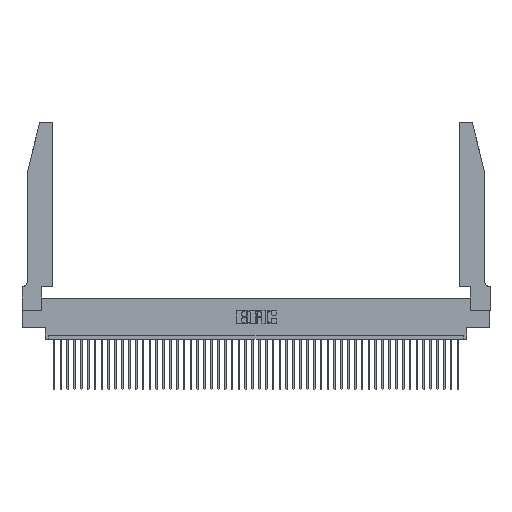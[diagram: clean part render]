
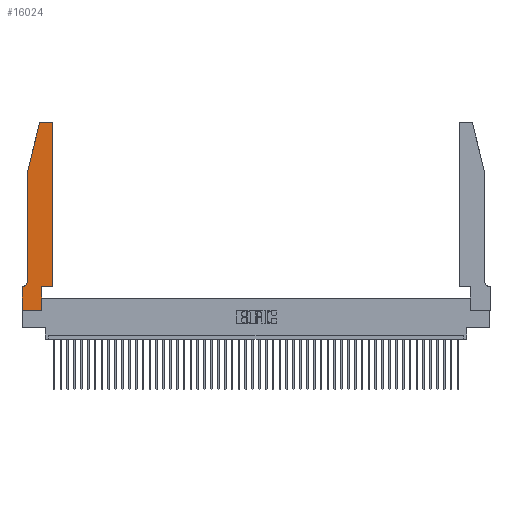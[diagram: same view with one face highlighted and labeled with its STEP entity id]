
A CAD part, top view. The second image highlights one B-rep face of the part: STEP entity #16024.
In plain terms, the highlighted planar face has unit normal (0, 0, 1).
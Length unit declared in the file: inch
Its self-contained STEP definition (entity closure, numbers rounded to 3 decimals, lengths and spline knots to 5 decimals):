
#218 = EDGE_CURVE ( 'NONE', #32804, #10812, #25990, .T. ) ;
#395 = VECTOR ( 'NONE', #32074, 39.37008 ) ;
#1540 = CARTESIAN_POINT ( 'NONE',  ( 0.284, 2.72, 0.37 ) ) ;
#2363 = VERTEX_POINT ( 'NONE', #44291 ) ;
#3165 = EDGE_CURVE ( 'NONE', #10812, #23474, #43766, .T. ) ;
#3370 = EDGE_CURVE ( 'NONE', #2363, #41579, #29880, .T. ) ;
#3627 = CARTESIAN_POINT ( 'NONE',  ( 0.2865, 0.35, 0.37 ) ) ;
#4248 = DIRECTION ( 'NONE',  ( 1., 0., 0. ) ) ;
#4582 = CARTESIAN_POINT ( 'NONE',  ( 0.4205, 2.72, 0.37 ) ) ;
#5202 = DIRECTION ( 'NONE',  ( 1., 0., 0. ) ) ;
#5893 = VECTOR ( 'NONE', #5202, 39.37008 ) ;
#6451 = LINE ( 'NONE', #23495, #5893 ) ;
#6571 = DIRECTION ( 'NONE',  ( 1., 0., 0. ) ) ;
#6599 = ORIENTED_EDGE ( 'NONE', *, *, #39795, .T. ) ;
#7477 = CARTESIAN_POINT ( 'NONE',  ( 0.0755, 0.35, 0.37 ) ) ;
#7932 = AXIS2_PLACEMENT_3D ( 'NONE', #4582, #29651, #4248 ) ;
#8199 = CIRCLE ( 'NONE', #40927, 0.03 ) ;
#8455 = ORIENTED_EDGE ( 'NONE', *, *, #41317, .T. ) ;
#9290 = DIRECTION ( 'NONE',  ( 0., 1., 0. ) ) ;
#9358 = VECTOR ( 'NONE', #35847, 39.37008 ) ;
#9424 = DIRECTION ( 'NONE',  ( 0., 0., -1. ) ) ;
#10183 = CARTESIAN_POINT ( 'NONE',  ( 0., 0., 0.37 ) ) ;
#10416 = DIRECTION ( 'NONE',  ( 0., 0., 1. ) ) ;
#10540 = CARTESIAN_POINT ( 'NONE',  ( 0.4505, 0.35, 0.37 ) ) ;
#10689 = EDGE_CURVE ( 'NONE', #14827, #32804, #16298, .T. ) ;
#10812 = VERTEX_POINT ( 'NONE', #33118 ) ;
#10949 = EDGE_CURVE ( 'NONE', #30766, #11461, #6451, .T. ) ;
#11461 = VERTEX_POINT ( 'NONE', #38514 ) ;
#12972 = DIRECTION ( 'NONE',  ( 1., 0., 0. ) ) ;
#13378 = EDGE_CURVE ( 'NONE', #41579, #30766, #16017, .T. ) ;
#13802 = CARTESIAN_POINT ( 'NONE',  ( 0.25487, 2.72718, 0.37 ) ) ;
#14827 = VERTEX_POINT ( 'NONE', #33170 ) ;
#15668 = CARTESIAN_POINT ( 'NONE',  ( 0., 0.35, 0.37 ) ) ;
#15968 = ORIENTED_EDGE ( 'NONE', *, *, #20642, .T. ) ;
#16017 = LINE ( 'NONE', #10183, #395 ) ;
#16024 = ADVANCED_FACE ( 'NONE', ( #43329 ), #28754, .T. ) ;
#16133 = VECTOR ( 'NONE', #38576, 39.37008 ) ;
#16298 = LINE ( 'NONE', #21199, #9358 ) ;
#17024 = ORIENTED_EDGE ( 'NONE', *, *, #21198, .T. ) ;
#17577 = ORIENTED_EDGE ( 'NONE', *, *, #218, .T. ) ;
#18183 = VERTEX_POINT ( 'NONE', #3627 ) ;
#18565 = DIRECTION ( 'NONE',  ( 1., 0., 0. ) ) ;
#18813 = ORIENTED_EDGE ( 'NONE', *, *, #10949, .T. ) ;
#18984 = CARTESIAN_POINT ( 'NONE',  ( 0.4505, 2.72, 0.37 ) ) ;
#19610 = CARTESIAN_POINT ( 'NONE',  ( 0.284, 2.75, 0.37 ) ) ;
#20233 = ORIENTED_EDGE ( 'NONE', *, *, #27962, .T. ) ;
#20393 = VERTEX_POINT ( 'NONE', #34395 ) ;
#20642 = EDGE_CURVE ( 'NONE', #20393, #34074, #46243, .T. ) ;
#21198 = EDGE_CURVE ( 'NONE', #34074, #2363, #28357, .T. ) ;
#21199 = CARTESIAN_POINT ( 'NONE',  ( 0.4505, 0.35, 0.37 ) ) ;
#22990 = VECTOR ( 'NONE', #31357, 39.37008 ) ;
#23200 = CARTESIAN_POINT ( 'NONE',  ( 0., 0., 0.37 ) ) ;
#23474 = VERTEX_POINT ( 'NONE', #19610 ) ;
#23495 = CARTESIAN_POINT ( 'NONE',  ( 0., 0., 0.37 ) ) ;
#23557 = LINE ( 'NONE', #46716, #16133 ) ;
#23791 = CARTESIAN_POINT ( 'NONE',  ( 0.2605, 2.75, 0.37 ) ) ;
#24556 = ORIENTED_EDGE ( 'NONE', *, *, #31477, .T. ) ;
#24865 = VERTEX_POINT ( 'NONE', #13802 ) ;
#24999 = VECTOR ( 'NONE', #9290, 39.37008 ) ;
#25050 = CARTESIAN_POINT ( 'NONE',  ( 0., 0.35, 0.37 ) ) ;
#25517 = VECTOR ( 'NONE', #40027, 39.37008 ) ;
#25990 = CIRCLE ( 'NONE', #7932, 0.03 ) ;
#27962 = EDGE_CURVE ( 'NONE', #24865, #20393, #23557, .T. ) ;
#28357 = CIRCLE ( 'NONE', #34177, 0.07 ) ;
#28754 = PLANE ( 'NONE',  #30347 ) ;
#29207 = CARTESIAN_POINT ( 'NONE',  ( 0.0755, 2., 0.37 ) ) ;
#29651 = DIRECTION ( 'NONE',  ( 0., 0., 1. ) ) ;
#29818 = CARTESIAN_POINT ( 'NONE',  ( 0.0755, 0.42, 0.37 ) ) ;
#29880 = LINE ( 'NONE', #7477, #45447 ) ;
#30347 = AXIS2_PLACEMENT_3D ( 'NONE', #25050, #10416, #6571 ) ;
#30401 = ORIENTED_EDGE ( 'NONE', *, *, #13378, .T. ) ;
#30766 = VERTEX_POINT ( 'NONE', #23200 ) ;
#31108 = DIRECTION ( 'NONE',  ( -1., 0., 0. ) ) ;
#31357 = DIRECTION ( 'NONE',  ( -1., 0., 0. ) ) ;
#31435 = CARTESIAN_POINT ( 'NONE',  ( 0.0055, 0.42, 0.37 ) ) ;
#31477 = EDGE_CURVE ( 'NONE', #23474, #24865, #8199, .T. ) ;
#32074 = DIRECTION ( 'NONE',  ( 0., -1., 0. ) ) ;
#32804 = VERTEX_POINT ( 'NONE', #18984 ) ;
#32832 = EDGE_LOOP ( 'NONE', ( #45989, #24556, #20233, #15968, #17024, #42349, #30401, #18813, #6599, #8455, #33730, #17577 ) ) ;
#33118 = CARTESIAN_POINT ( 'NONE',  ( 0.4205, 2.75, 0.37 ) ) ;
#33170 = CARTESIAN_POINT ( 'NONE',  ( 0.4505, 0.35, 0.37 ) ) ;
#33655 = DIRECTION ( 'NONE',  ( -1., 0., 0. ) ) ;
#33730 = ORIENTED_EDGE ( 'NONE', *, *, #10689, .T. ) ;
#34074 = VERTEX_POINT ( 'NONE', #29818 ) ;
#34177 = AXIS2_PLACEMENT_3D ( 'NONE', #31435, #9424, #31108 ) ;
#34395 = CARTESIAN_POINT ( 'NONE',  ( 0.0755, 2., 0.37 ) ) ;
#34581 = VECTOR ( 'NONE', #18565, 39.37008 ) ;
#35847 = DIRECTION ( 'NONE',  ( 0., 1., 0. ) ) ;
#38514 = CARTESIAN_POINT ( 'NONE',  ( 0.2865, 0., 0.37 ) ) ;
#38527 = DIRECTION ( 'NONE',  ( 0., 0., 1. ) ) ;
#38554 = CARTESIAN_POINT ( 'NONE',  ( 0.2865, 0.35, 0.37 ) ) ;
#38576 = DIRECTION ( 'NONE',  ( -0.239, -0.971, 0. ) ) ;
#39418 = LINE ( 'NONE', #38554, #24999 ) ;
#39795 = EDGE_CURVE ( 'NONE', #11461, #18183, #39418, .T. ) ;
#40027 = DIRECTION ( 'NONE',  ( 0., -1., 0. ) ) ;
#40927 = AXIS2_PLACEMENT_3D ( 'NONE', #1540, #38527, #12972 ) ;
#41317 = EDGE_CURVE ( 'NONE', #18183, #14827, #44320, .T. ) ;
#41579 = VERTEX_POINT ( 'NONE', #15668 ) ;
#42349 = ORIENTED_EDGE ( 'NONE', *, *, #3370, .T. ) ;
#43329 = FACE_OUTER_BOUND ( 'NONE', #32832, .T. ) ;
#43766 = LINE ( 'NONE', #23791, #22990 ) ;
#44291 = CARTESIAN_POINT ( 'NONE',  ( 0.0055, 0.35, 0.37 ) ) ;
#44320 = LINE ( 'NONE', #10540, #34581 ) ;
#45447 = VECTOR ( 'NONE', #33655, 39.37008 ) ;
#45989 = ORIENTED_EDGE ( 'NONE', *, *, #3165, .T. ) ;
#46243 = LINE ( 'NONE', #29207, #25517 ) ;
#46716 = CARTESIAN_POINT ( 'NONE',  ( 0.0755, 2., 0.37 ) ) ;
